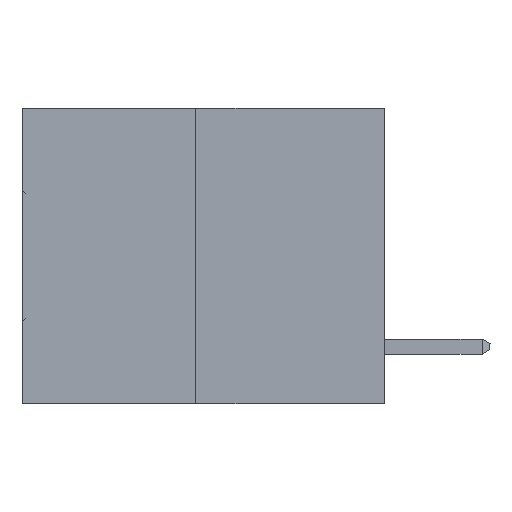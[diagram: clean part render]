
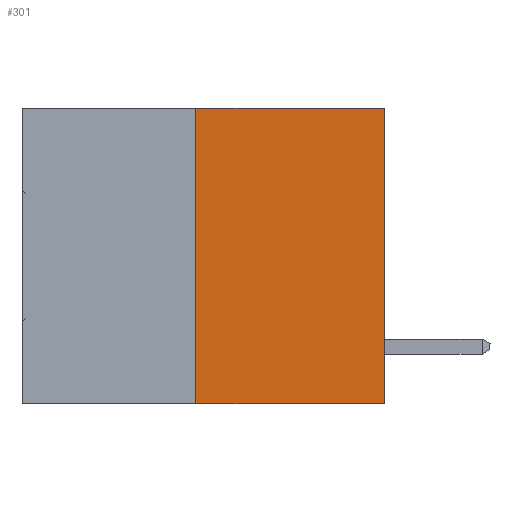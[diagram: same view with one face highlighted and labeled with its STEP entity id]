
A CAD part, left-side view. The second image highlights one B-rep face of the part: STEP entity #301.
In plain terms, the highlighted planar face has unit normal (-1, 0, 0).
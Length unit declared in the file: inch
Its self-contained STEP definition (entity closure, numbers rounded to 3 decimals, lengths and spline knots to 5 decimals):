
#184 = DIRECTION ( 'NONE',  ( 0., 0., 1. ) ) ;
#301 = ADVANCED_FACE ( 'NONE', ( #18757 ), #27634, .F. ) ;
#1085 = ORIENTED_EDGE ( 'NONE', *, *, #17664, .T. ) ;
#1622 = VERTEX_POINT ( 'NONE', #7437 ) ;
#2294 = CARTESIAN_POINT ( 'NONE',  ( 0., 0., 0. ) ) ;
#3435 = DIRECTION ( 'NONE',  ( 0., -1., 0. ) ) ;
#7287 = DIRECTION ( 'NONE',  ( 0., -1., 0. ) ) ;
#7437 = CARTESIAN_POINT ( 'NONE',  ( 0., 0.312, 0. ) ) ;
#9079 = CARTESIAN_POINT ( 'NONE',  ( 0., 0., -0.49 ) ) ;
#9109 = AXIS2_PLACEMENT_3D ( 'NONE', #35423, #24446, #12871 ) ;
#9315 = VERTEX_POINT ( 'NONE', #9079 ) ;
#10370 = VERTEX_POINT ( 'NONE', #13456 ) ;
#12147 = ORIENTED_EDGE ( 'NONE', *, *, #21708, .F. ) ;
#12386 = VECTOR ( 'NONE', #184, 39.37008 ) ;
#12871 = DIRECTION ( 'NONE',  ( 0., 0., -1. ) ) ;
#13456 = CARTESIAN_POINT ( 'NONE',  ( 0., 0.312, -0.49 ) ) ;
#13746 = VECTOR ( 'NONE', #3435, 39.37008 ) ;
#14124 = CARTESIAN_POINT ( 'NONE',  ( 0., 0., 0. ) ) ;
#14374 = VECTOR ( 'NONE', #19863, 39.37008 ) ;
#17664 = EDGE_CURVE ( 'NONE', #9315, #21985, #21449, .T. ) ;
#18757 = FACE_OUTER_BOUND ( 'NONE', #18866, .T. ) ;
#18866 = EDGE_LOOP ( 'NONE', ( #33323, #30110, #1085, #12147 ) ) ;
#19863 = DIRECTION ( 'NONE',  ( 0., 0., 1. ) ) ;
#20654 = LINE ( 'NONE', #29170, #27345 ) ;
#21449 = LINE ( 'NONE', #14124, #12386 ) ;
#21514 = LINE ( 'NONE', #33836, #13746 ) ;
#21708 = EDGE_CURVE ( 'NONE', #1622, #21985, #21514, .T. ) ;
#21985 = VERTEX_POINT ( 'NONE', #2294 ) ;
#22583 = LINE ( 'NONE', #28168, #14374 ) ;
#24446 = DIRECTION ( 'NONE',  ( 1., 0., 0. ) ) ;
#27345 = VECTOR ( 'NONE', #7287, 39.37008 ) ;
#27634 = PLANE ( 'NONE',  #9109 ) ;
#28168 = CARTESIAN_POINT ( 'NONE',  ( 0., 0.312, -0.49 ) ) ;
#28712 = EDGE_CURVE ( 'NONE', #10370, #9315, #20654, .T. ) ;
#29170 = CARTESIAN_POINT ( 'NONE',  ( 0., 0.6, -0.49 ) ) ;
#30110 = ORIENTED_EDGE ( 'NONE', *, *, #28712, .T. ) ;
#33323 = ORIENTED_EDGE ( 'NONE', *, *, #35263, .F. ) ;
#33836 = CARTESIAN_POINT ( 'NONE',  ( 0., 0.6, 0. ) ) ;
#35263 = EDGE_CURVE ( 'NONE', #10370, #1622, #22583, .T. ) ;
#35423 = CARTESIAN_POINT ( 'NONE',  ( 0., 0.6, 0. ) ) ;
